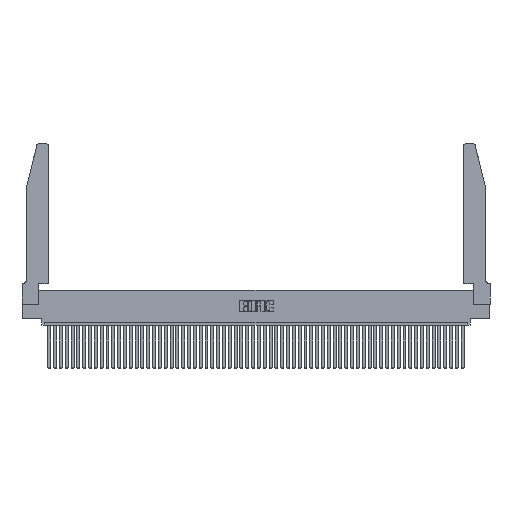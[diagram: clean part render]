
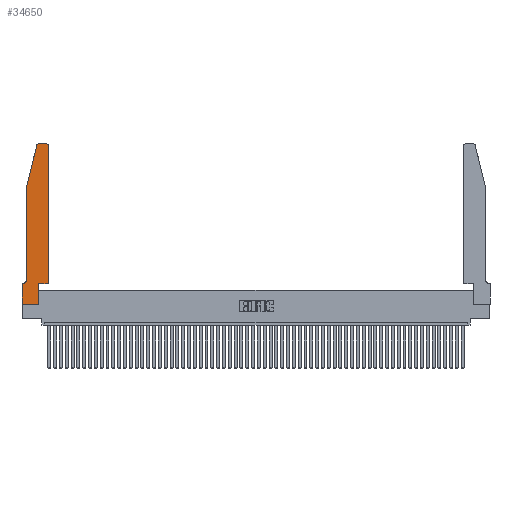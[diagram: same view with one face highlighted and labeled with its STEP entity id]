
A CAD part, top view. The second image highlights one B-rep face of the part: STEP entity #34650.
In plain terms, the highlighted planar face has unit normal (0, 0, 1).
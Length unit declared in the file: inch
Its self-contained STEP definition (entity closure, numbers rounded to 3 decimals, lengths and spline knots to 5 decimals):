
#60 = VECTOR ( 'NONE', #5378, 39.37008 ) ;
#446 = CARTESIAN_POINT ( 'NONE',  ( 0.4505, 0.35, 0.37 ) ) ;
#1873 = EDGE_CURVE ( 'NONE', #6695, #49914, #24233, .T. ) ;
#2289 = CIRCLE ( 'NONE', #10335, 0.07 ) ;
#2744 = CARTESIAN_POINT ( 'NONE',  ( 0.25487, 2.72718, 0.37 ) ) ;
#3346 = CARTESIAN_POINT ( 'NONE',  ( 0.2865, 0.35, 0.37 ) ) ;
#3434 = CARTESIAN_POINT ( 'NONE',  ( 0., 0., 0.37 ) ) ;
#3763 = VECTOR ( 'NONE', #54066, 39.37008 ) ;
#3846 = DIRECTION ( 'NONE',  ( -1., 0., 0. ) ) ;
#5378 = DIRECTION ( 'NONE',  ( 1., 0., 0. ) ) ;
#6356 = DIRECTION ( 'NONE',  ( 0., 1., 0. ) ) ;
#6566 = VECTOR ( 'NONE', #8875, 39.37008 ) ;
#6695 = VERTEX_POINT ( 'NONE', #29175 ) ;
#6733 = CARTESIAN_POINT ( 'NONE',  ( 0.4505, 0.35, 0.37 ) ) ;
#6965 = ORIENTED_EDGE ( 'NONE', *, *, #14068, .T. ) ;
#7604 = DIRECTION ( 'NONE',  ( 0., 1., 0. ) ) ;
#7711 = EDGE_CURVE ( 'NONE', #31653, #22436, #43615, .T. ) ;
#8464 = DIRECTION ( 'NONE',  ( 0., 0., 1. ) ) ;
#8875 = DIRECTION ( 'NONE',  ( 0., -1., 0. ) ) ;
#9016 = VECTOR ( 'NONE', #7604, 39.37008 ) ;
#9736 = DIRECTION ( 'NONE',  ( 1., 0., 0. ) ) ;
#10335 = AXIS2_PLACEMENT_3D ( 'NONE', #49586, #53874, #24280 ) ;
#10706 = DIRECTION ( 'NONE',  ( -1., 0., 0. ) ) ;
#11944 = VERTEX_POINT ( 'NONE', #40559 ) ;
#12013 = EDGE_CURVE ( 'NONE', #20458, #20406, #15132, .T. ) ;
#12830 = LINE ( 'NONE', #36231, #23449 ) ;
#13131 = CARTESIAN_POINT ( 'NONE',  ( 0., 0., 0.37 ) ) ;
#13197 = LINE ( 'NONE', #6733, #28486 ) ;
#13548 = EDGE_CURVE ( 'NONE', #49914, #20458, #30275, .T. ) ;
#14068 = EDGE_CURVE ( 'NONE', #37701, #46340, #46055, .T. ) ;
#14551 = ORIENTED_EDGE ( 'NONE', *, *, #20532, .T. ) ;
#14949 = ORIENTED_EDGE ( 'NONE', *, *, #47582, .T. ) ;
#15132 = LINE ( 'NONE', #29987, #6566 ) ;
#15145 = VECTOR ( 'NONE', #54211, 39.37008 ) ;
#17815 = VERTEX_POINT ( 'NONE', #3434 ) ;
#18843 = CARTESIAN_POINT ( 'NONE',  ( 0.0755, 0.35, 0.37 ) ) ;
#20235 = EDGE_LOOP ( 'NONE', ( #14551, #40020, #35346, #29396, #32031, #6965, #40269, #31739, #14949, #35735, #46009, #34081 ) ) ;
#20406 = VERTEX_POINT ( 'NONE', #24216 ) ;
#20458 = VERTEX_POINT ( 'NONE', #24957 ) ;
#20532 = EDGE_CURVE ( 'NONE', #28962, #6695, #53570, .T. ) ;
#21223 = LINE ( 'NONE', #13131, #60 ) ;
#22037 = CARTESIAN_POINT ( 'NONE',  ( 0.4205, 2.75, 0.37 ) ) ;
#22436 = VERTEX_POINT ( 'NONE', #446 ) ;
#22499 = CARTESIAN_POINT ( 'NONE',  ( 0., 0.35, 0.37 ) ) ;
#23449 = VECTOR ( 'NONE', #35854, 39.37008 ) ;
#24216 = CARTESIAN_POINT ( 'NONE',  ( 0.0755, 0.42, 0.37 ) ) ;
#24233 = CIRCLE ( 'NONE', #53787, 0.03 ) ;
#24280 = DIRECTION ( 'NONE',  ( -1., 0., 0. ) ) ;
#24434 = VECTOR ( 'NONE', #3846, 39.37008 ) ;
#24437 = CARTESIAN_POINT ( 'NONE',  ( 0.4505, 0.35, 0.37 ) ) ;
#24474 = CARTESIAN_POINT ( 'NONE',  ( 0.2865, 0.35, 0.37 ) ) ;
#24957 = CARTESIAN_POINT ( 'NONE',  ( 0.0755, 2., 0.37 ) ) ;
#28486 = VECTOR ( 'NONE', #6356, 39.37008 ) ;
#28642 = VERTEX_POINT ( 'NONE', #35752 ) ;
#28962 = VERTEX_POINT ( 'NONE', #22037 ) ;
#28984 = CARTESIAN_POINT ( 'NONE',  ( 0.0055, 0.35, 0.37 ) ) ;
#29175 = CARTESIAN_POINT ( 'NONE',  ( 0.284, 2.75, 0.37 ) ) ;
#29226 = CARTESIAN_POINT ( 'NONE',  ( 0.2605, 2.75, 0.37 ) ) ;
#29396 = ORIENTED_EDGE ( 'NONE', *, *, #12013, .T. ) ;
#29987 = CARTESIAN_POINT ( 'NONE',  ( 0.0755, 2., 0.37 ) ) ;
#30275 = LINE ( 'NONE', #53693, #3763 ) ;
#31653 = VERTEX_POINT ( 'NONE', #3346 ) ;
#31739 = ORIENTED_EDGE ( 'NONE', *, *, #36841, .T. ) ;
#32031 = ORIENTED_EDGE ( 'NONE', *, *, #45455, .T. ) ;
#34081 = ORIENTED_EDGE ( 'NONE', *, *, #37230, .T. ) ;
#34374 = CARTESIAN_POINT ( 'NONE',  ( 0., 0.35, 0.37 ) ) ;
#34650 = ADVANCED_FACE ( 'NONE', ( #53314 ), #34890, .T. ) ;
#34890 = PLANE ( 'NONE',  #44009 ) ;
#35251 = DIRECTION ( 'NONE',  ( 0., 0., 1. ) ) ;
#35346 = ORIENTED_EDGE ( 'NONE', *, *, #13548, .T. ) ;
#35735 = ORIENTED_EDGE ( 'NONE', *, *, #7711, .T. ) ;
#35752 = CARTESIAN_POINT ( 'NONE',  ( 0.4505, 2.72, 0.37 ) ) ;
#35854 = DIRECTION ( 'NONE',  ( 0., -1., 0. ) ) ;
#36231 = CARTESIAN_POINT ( 'NONE',  ( 0., 0., 0.37 ) ) ;
#36841 = EDGE_CURVE ( 'NONE', #17815, #11944, #21223, .T. ) ;
#37096 = CIRCLE ( 'NONE', #45175, 0.03 ) ;
#37230 = EDGE_CURVE ( 'NONE', #28642, #28962, #37096, .T. ) ;
#37337 = CARTESIAN_POINT ( 'NONE',  ( 0.4205, 2.72, 0.37 ) ) ;
#37701 = VERTEX_POINT ( 'NONE', #28984 ) ;
#38146 = EDGE_CURVE ( 'NONE', #22436, #28642, #13197, .T. ) ;
#39728 = CARTESIAN_POINT ( 'NONE',  ( 0.284, 2.72, 0.37 ) ) ;
#39919 = DIRECTION ( 'NONE',  ( 1., 0., 0. ) ) ;
#40020 = ORIENTED_EDGE ( 'NONE', *, *, #1873, .T. ) ;
#40269 = ORIENTED_EDGE ( 'NONE', *, *, #46081, .T. ) ;
#40559 = CARTESIAN_POINT ( 'NONE',  ( 0.2865, 0., 0.37 ) ) ;
#40740 = LINE ( 'NONE', #24474, #9016 ) ;
#41595 = DIRECTION ( 'NONE',  ( 1., 0., 0. ) ) ;
#42062 = VECTOR ( 'NONE', #10706, 39.37008 ) ;
#43615 = LINE ( 'NONE', #24437, #15145 ) ;
#44009 = AXIS2_PLACEMENT_3D ( 'NONE', #22499, #35251, #9736 ) ;
#45175 = AXIS2_PLACEMENT_3D ( 'NONE', #37337, #8464, #41595 ) ;
#45455 = EDGE_CURVE ( 'NONE', #20406, #37701, #2289, .T. ) ;
#46009 = ORIENTED_EDGE ( 'NONE', *, *, #38146, .T. ) ;
#46055 = LINE ( 'NONE', #18843, #42062 ) ;
#46081 = EDGE_CURVE ( 'NONE', #46340, #17815, #12830, .T. ) ;
#46340 = VERTEX_POINT ( 'NONE', #34374 ) ;
#47582 = EDGE_CURVE ( 'NONE', #11944, #31653, #40740, .T. ) ;
#48230 = DIRECTION ( 'NONE',  ( 0., 0., 1. ) ) ;
#49586 = CARTESIAN_POINT ( 'NONE',  ( 0.0055, 0.42, 0.37 ) ) ;
#49914 = VERTEX_POINT ( 'NONE', #2744 ) ;
#53314 = FACE_OUTER_BOUND ( 'NONE', #20235, .T. ) ;
#53570 = LINE ( 'NONE', #29226, #24434 ) ;
#53693 = CARTESIAN_POINT ( 'NONE',  ( 0.0755, 2., 0.37 ) ) ;
#53787 = AXIS2_PLACEMENT_3D ( 'NONE', #39728, #48230, #39919 ) ;
#53874 = DIRECTION ( 'NONE',  ( 0., 0., -1. ) ) ;
#54066 = DIRECTION ( 'NONE',  ( -0.239, -0.971, 0. ) ) ;
#54211 = DIRECTION ( 'NONE',  ( 1., 0., 0. ) ) ;
